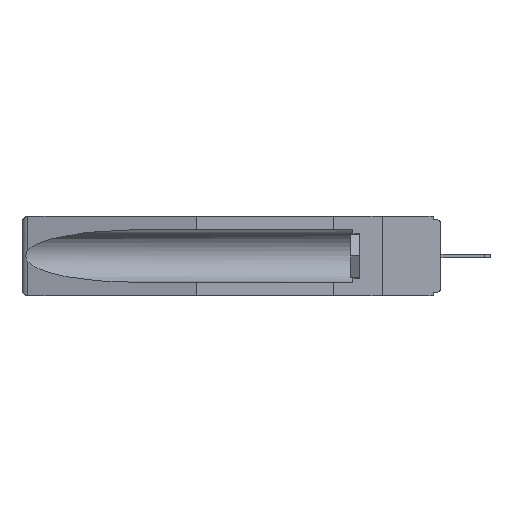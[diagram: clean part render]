
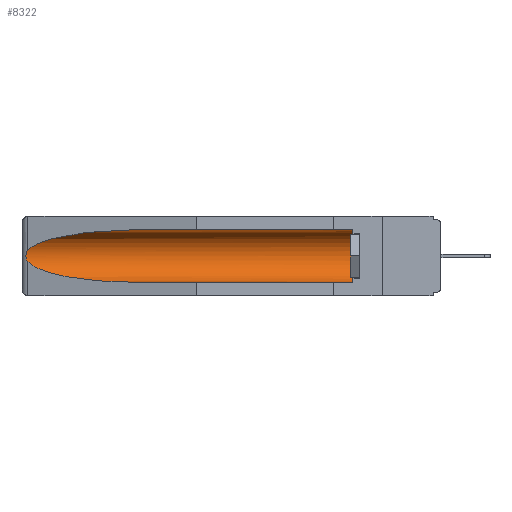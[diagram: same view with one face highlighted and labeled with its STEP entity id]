
A CAD part, left-side view. The second image highlights one B-rep face of the part: STEP entity #8322.
In plain terms, the highlighted cylindrical face has radius 2.857 mm (diameter 5.715 mm), a partial arc.
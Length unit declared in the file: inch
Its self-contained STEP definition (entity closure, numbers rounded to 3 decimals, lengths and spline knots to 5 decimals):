
#372 = CARTESIAN_POINT ( 'NONE',  ( 0.155, 1.07973, -0.059 ) ) ;
#577 = CARTESIAN_POINT ( 'NONE',  ( 0.26597, 1.52961, -0.15275 ) ) ;
#672 = CARTESIAN_POINT ( 'NONE',  ( 0.26537, 1.52718, -0.19328 ) ) ;
#825 = DIRECTION ( 'NONE',  ( 0., 0., 1. ) ) ;
#1227 = ORIENTED_EDGE ( 'NONE', *, *, #13369, .T. ) ;
#1422 = VERTEX_POINT ( 'NONE', #13637 ) ;
#1828 = CARTESIAN_POINT ( 'NONE',  ( 0.26655, 1.53094, -0.18657 ) ) ;
#2099 = CARTESIAN_POINT ( 'NONE',  ( 0.21114, 1.30732, -0.284 ) ) ;
#2564 = CARTESIAN_POINT ( 'NONE',  ( 0.155, 0.126, -0.284 ) ) ;
#2662 = CARTESIAN_POINT ( 'NONE',  ( 0.26537, 1.52718, -0.14972 ) ) ;
#2856 = DIRECTION ( 'NONE',  ( 0., 1., 0. ) ) ;
#2911 = DIRECTION ( 'NONE',  ( 0., 0., 1. ) ) ;
#2990 = FACE_OUTER_BOUND ( 'NONE', #14803, .T. ) ;
#3032 = EDGE_CURVE ( 'NONE', #1422, #15445, #5502, .T. ) ;
#3126 =( BOUNDED_CURVE ( )  B_SPLINE_CURVE ( 3, ( #9111, #17310, #8049, #5205 ),
 .UNSPECIFIED., .F., .T. ) 
 B_SPLINE_CURVE_WITH_KNOTS ( ( 4, 4 ),
 ( 4.71239, 6.08839 ),
 .UNSPECIFIED. ) 
 CURVE ( )  GEOMETRIC_REPRESENTATION_ITEM ( )  RATIONAL_B_SPLINE_CURVE ( ( 1., 0.848, 0.848, 1. ) ) 
 REPRESENTATION_ITEM ( '' )  );
#3315 = AXIS2_PLACEMENT_3D ( 'NONE', #9636, #16447, #2911 ) ;
#3328 = EDGE_CURVE ( 'NONE', #9353, #9825, #16348, .T. ) ;
#4021 = LINE ( 'NONE', #15041, #11421 ) ;
#4132 = CARTESIAN_POINT ( 'NONE',  ( 0.155, 0.126, -0.059 ) ) ;
#4158 = ORIENTED_EDGE ( 'NONE', *, *, #3328, .T. ) ;
#4239 = CYLINDRICAL_SURFACE ( 'NONE', #3315, 0.1125 ) ;
#4392 = EDGE_CURVE ( 'NONE', #11949, #1422, #11466, .T. ) ;
#4405 = CARTESIAN_POINT ( 'NONE',  ( 0.2673, 1.53269, -0.17917 ) ) ;
#4849 = CARTESIAN_POINT ( 'NONE',  ( 0.25451, 1.48313, -0.24835 ) ) ;
#4949 = CARTESIAN_POINT ( 'NONE',  ( 0.155, -0.30754, -0.059 ) ) ;
#5103 = CARTESIAN_POINT ( 'NONE',  ( 0.155, 1.07973, -0.284 ) ) ;
#5205 = CARTESIAN_POINT ( 'NONE',  ( 0.26537, 1.52718, -0.14972 ) ) ;
#5502 =( BOUNDED_CURVE ( )  B_SPLINE_CURVE ( 3, ( #672, #4849, #2099, #5103 ),
 .UNSPECIFIED., .F., .T. ) 
 B_SPLINE_CURVE_WITH_KNOTS ( ( 4, 4 ),
 ( 0.1948, 1.5708 ),
 .UNSPECIFIED. ) 
 CURVE ( )  GEOMETRIC_REPRESENTATION_ITEM ( )  RATIONAL_B_SPLINE_CURVE ( ( 1., 0.848, 0.848, 1. ) ) 
 REPRESENTATION_ITEM ( '' )  );
#5639 = EDGE_CURVE ( 'NONE', #7829, #11949, #3126, .T. ) ;
#5748 = CARTESIAN_POINT ( 'NONE',  ( 0.2673, 1.5327, -0.16383 ) ) ;
#5997 = CARTESIAN_POINT ( 'NONE',  ( 0.2675, 1.53308, -0.17534 ) ) ;
#6072 = EDGE_CURVE ( 'NONE', #9353, #15445, #4021, .T. ) ;
#6979 = CARTESIAN_POINT ( 'NONE',  ( 0.26597, 1.5296, -0.19026 ) ) ;
#7062 = CARTESIAN_POINT ( 'NONE',  ( 0.2675, 1.53308, -0.16763 ) ) ;
#7705 = VECTOR ( 'NONE', #15803, 39.37008 ) ;
#7829 = VERTEX_POINT ( 'NONE', #372 ) ;
#8049 = CARTESIAN_POINT ( 'NONE',  ( 0.25451, 1.48313, -0.09465 ) ) ;
#8322 = ADVANCED_FACE ( 'NONE', ( #2990 ), #4239, .F. ) ;
#8566 = CARTESIAN_POINT ( 'NONE',  ( 0.26654, 1.53092, -0.15636 ) ) ;
#9111 = CARTESIAN_POINT ( 'NONE',  ( 0.155, 1.07973, -0.059 ) ) ;
#9353 = VERTEX_POINT ( 'NONE', #2564 ) ;
#9636 = CARTESIAN_POINT ( 'NONE',  ( 0.155, -0.30754, -0.1715 ) ) ;
#9825 = VERTEX_POINT ( 'NONE', #4132 ) ;
#9966 = CARTESIAN_POINT ( 'NONE',  ( 0.26537, 1.52718, -0.19328 ) ) ;
#11421 = VECTOR ( 'NONE', #2856, 39.37008 ) ;
#11466 = B_SPLINE_CURVE_WITH_KNOTS ( 'NONE', 3,
 ( #14021, #577, #8566, #5748, #7062, #5997, #4405, #1828, #6979, #9966 ),
 .UNSPECIFIED., .F., .F.,
 ( 4, 2, 2, 2, 4 ),
 ( 0., 0.00029, 0.00058, 0.00087, 0.00117 ),
 .UNSPECIFIED. ) ;
#11931 = LINE ( 'NONE', #4949, #7705 ) ;
#11949 = VERTEX_POINT ( 'NONE', #2662 ) ;
#12642 = ORIENTED_EDGE ( 'NONE', *, *, #4392, .T. ) ;
#12782 = DIRECTION ( 'NONE',  ( 0., -1., 0. ) ) ;
#13369 = EDGE_CURVE ( 'NONE', #9825, #7829, #11931, .T. ) ;
#13637 = CARTESIAN_POINT ( 'NONE',  ( 0.26537, 1.52718, -0.19328 ) ) ;
#13680 = CARTESIAN_POINT ( 'NONE',  ( 0.155, 1.07973, -0.284 ) ) ;
#14021 = CARTESIAN_POINT ( 'NONE',  ( 0.26537, 1.52718, -0.14972 ) ) ;
#14803 = EDGE_LOOP ( 'NONE', ( #15524, #12642, #17170, #16954, #4158, #1227 ) ) ;
#15041 = CARTESIAN_POINT ( 'NONE',  ( 0.155, -0.30754, -0.284 ) ) ;
#15185 = AXIS2_PLACEMENT_3D ( 'NONE', #17017, #12782, #825 ) ;
#15445 = VERTEX_POINT ( 'NONE', #13680 ) ;
#15524 = ORIENTED_EDGE ( 'NONE', *, *, #5639, .T. ) ;
#15803 = DIRECTION ( 'NONE',  ( 0., 1., 0. ) ) ;
#16348 = CIRCLE ( 'NONE', #15185, 0.1125 ) ;
#16447 = DIRECTION ( 'NONE',  ( 0., 1., 0. ) ) ;
#16954 = ORIENTED_EDGE ( 'NONE', *, *, #6072, .F. ) ;
#17017 = CARTESIAN_POINT ( 'NONE',  ( 0.155, 0.126, -0.1715 ) ) ;
#17170 = ORIENTED_EDGE ( 'NONE', *, *, #3032, .T. ) ;
#17310 = CARTESIAN_POINT ( 'NONE',  ( 0.21114, 1.30732, -0.059 ) ) ;
